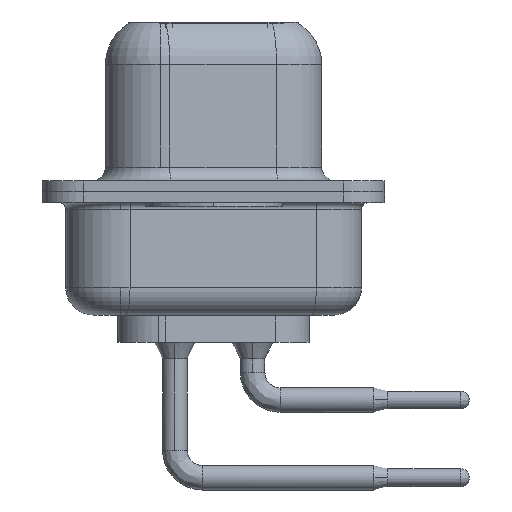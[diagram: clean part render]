
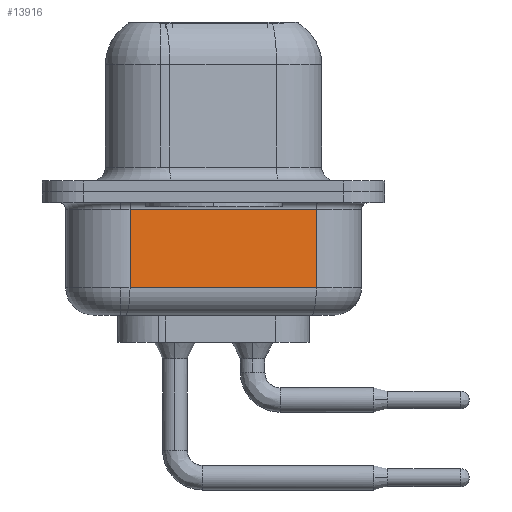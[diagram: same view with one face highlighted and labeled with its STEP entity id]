
A CAD part, left-side view. The second image highlights one B-rep face of the part: STEP entity #13916.
In plain terms, the highlighted planar face has unit normal (-0.985, -0.174, 0).
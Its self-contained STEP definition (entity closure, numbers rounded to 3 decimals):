
#167 = AXIS2_PLACEMENT_3D ( 'NONE', #1312, #16863, #7627 ) ;
#888 = CARTESIAN_POINT ( 'NONE',  ( 4.054, -3.747, -4.5 ) ) ;
#1263 = CARTESIAN_POINT ( 'NONE',  ( 2.855, 3.053, -0.65 ) ) ;
#1312 = CARTESIAN_POINT ( 'NONE',  ( 2.855, 3.053, -4.5 ) ) ;
#1640 = CARTESIAN_POINT ( 'NONE',  ( 2.855, 3.053, -3.5 ) ) ;
#4082 = LINE ( 'NONE', #18026, #20072 ) ;
#4390 = LINE ( 'NONE', #1263, #12645 ) ;
#4817 = VERTEX_POINT ( 'NONE', #1640 ) ;
#5396 = ORIENTED_EDGE ( 'NONE', *, *, #8015, .T. ) ;
#6079 = PLANE ( 'NONE',  #167 ) ;
#7627 = DIRECTION ( 'NONE',  ( -0.174, 0.985, 0. ) ) ;
#7657 = LINE ( 'NONE', #16526, #11314 ) ;
#8015 = EDGE_CURVE ( 'NONE', #13656, #8089, #15221, .T. ) ;
#8089 = VERTEX_POINT ( 'NONE', #19450 ) ;
#8239 = EDGE_CURVE ( 'NONE', #4817, #10112, #4082, .T. ) ;
#10112 = VERTEX_POINT ( 'NONE', #11057 ) ;
#11057 = CARTESIAN_POINT ( 'NONE',  ( 2.855, 3.053, -0.65 ) ) ;
#11170 = VECTOR ( 'NONE', #11844, 1000. ) ;
#11314 = VECTOR ( 'NONE', #18101, 1000. ) ;
#11844 = DIRECTION ( 'NONE',  ( 0., 0., 1. ) ) ;
#12645 = VECTOR ( 'NONE', #19878, 1000. ) ;
#13656 = VERTEX_POINT ( 'NONE', #19322 ) ;
#13916 = ADVANCED_FACE ( 'NONE', ( #19695 ), #6079, .F. ) ;
#14737 = EDGE_LOOP ( 'NONE', ( #17587, #16837, #5396, #18847 ) ) ;
#15099 = EDGE_CURVE ( 'NONE', #8089, #10112, #4390, .T. ) ;
#15221 = LINE ( 'NONE', #888, #11170 ) ;
#16526 = CARTESIAN_POINT ( 'NONE',  ( 2.855, 3.053, -3.5 ) ) ;
#16837 = ORIENTED_EDGE ( 'NONE', *, *, #18455, .T. ) ;
#16863 = DIRECTION ( 'NONE',  ( 0.985, 0.174, 0. ) ) ;
#17587 = ORIENTED_EDGE ( 'NONE', *, *, #8239, .F. ) ;
#18026 = CARTESIAN_POINT ( 'NONE',  ( 2.855, 3.053, -4.5 ) ) ;
#18087 = DIRECTION ( 'NONE',  ( 0., 0., 1. ) ) ;
#18101 = DIRECTION ( 'NONE',  ( 0.174, -0.985, 0. ) ) ;
#18455 = EDGE_CURVE ( 'NONE', #4817, #13656, #7657, .T. ) ;
#18847 = ORIENTED_EDGE ( 'NONE', *, *, #15099, .T. ) ;
#19322 = CARTESIAN_POINT ( 'NONE',  ( 4.054, -3.747, -3.5 ) ) ;
#19450 = CARTESIAN_POINT ( 'NONE',  ( 4.054, -3.747, -0.65 ) ) ;
#19695 = FACE_OUTER_BOUND ( 'NONE', #14737, .T. ) ;
#19878 = DIRECTION ( 'NONE',  ( -0.174, 0.985, 0. ) ) ;
#20072 = VECTOR ( 'NONE', #18087, 1000. ) ;
